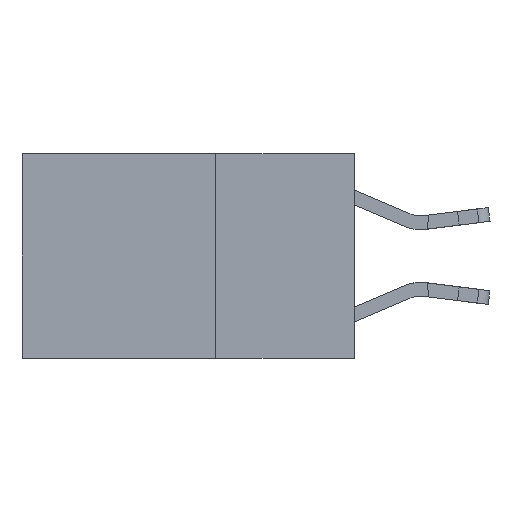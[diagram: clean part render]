
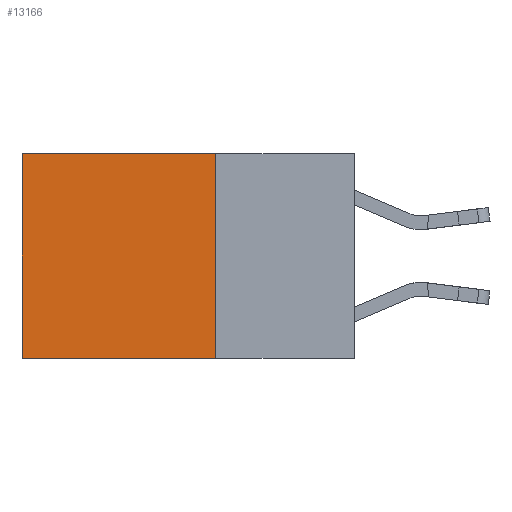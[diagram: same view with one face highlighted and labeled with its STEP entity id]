
A CAD part, left-side view. The second image highlights one B-rep face of the part: STEP entity #13166.
In plain terms, the highlighted planar face has unit normal (-1, 0, 0).
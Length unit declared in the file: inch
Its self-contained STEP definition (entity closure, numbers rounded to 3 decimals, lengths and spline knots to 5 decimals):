
#36 = EDGE_LOOP ( 'NONE', ( #1351, #12212, #3671, #1353 ) ) ;
#276 = FACE_OUTER_BOUND ( 'NONE', #36, .T. ) ;
#510 = DIRECTION ( 'NONE',  ( 0., 0., -1. ) ) ;
#727 = EDGE_CURVE ( 'NONE', #2902, #9760, #1967, .T. ) ;
#980 = VECTOR ( 'NONE', #510, 39.37008 ) ;
#1351 = ORIENTED_EDGE ( 'NONE', *, *, #727, .T. ) ;
#1353 = ORIENTED_EDGE ( 'NONE', *, *, #10405, .T. ) ;
#1362 = CARTESIAN_POINT ( 'NONE',  ( 0.2625, 0.25, 0. ) ) ;
#1462 = VERTEX_POINT ( 'NONE', #5205 ) ;
#1967 = LINE ( 'NONE', #6863, #980 ) ;
#2902 = VERTEX_POINT ( 'NONE', #10292 ) ;
#3411 = EDGE_CURVE ( 'NONE', #1462, #8836, #15473, .T. ) ;
#3662 = DIRECTION ( 'NONE',  ( 1., 0., 0. ) ) ;
#3671 = ORIENTED_EDGE ( 'NONE', *, *, #3411, .F. ) ;
#3880 = CARTESIAN_POINT ( 'NONE',  ( 0.2625, 0.25, -0.37 ) ) ;
#3924 = DIRECTION ( 'NONE',  ( 0., 1., 0. ) ) ;
#5205 = CARTESIAN_POINT ( 'NONE',  ( 0.2625, 0.25, 0. ) ) ;
#5768 = LINE ( 'NONE', #1362, #12105 ) ;
#6618 = CARTESIAN_POINT ( 'NONE',  ( 0.2625, 0.25, 0. ) ) ;
#6775 = DIRECTION ( 'NONE',  ( 0., 1., 0. ) ) ;
#6863 = CARTESIAN_POINT ( 'NONE',  ( 0.2625, 0.6, 0. ) ) ;
#8833 = DIRECTION ( 'NONE',  ( 0., 0., -1. ) ) ;
#8836 = VERTEX_POINT ( 'NONE', #3880 ) ;
#9350 = CARTESIAN_POINT ( 'NONE',  ( 0.2625, 0.6, -0.37 ) ) ;
#9760 = VERTEX_POINT ( 'NONE', #9350 ) ;
#10292 = CARTESIAN_POINT ( 'NONE',  ( 0.2625, 0.6, 0. ) ) ;
#10293 = VECTOR ( 'NONE', #14247, 39.37008 ) ;
#10302 = VECTOR ( 'NONE', #6775, 39.37008 ) ;
#10405 = EDGE_CURVE ( 'NONE', #1462, #2902, #5768, .T. ) ;
#11240 = EDGE_CURVE ( 'NONE', #8836, #9760, #13695, .T. ) ;
#12105 = VECTOR ( 'NONE', #3924, 39.37008 ) ;
#12212 = ORIENTED_EDGE ( 'NONE', *, *, #11240, .F. ) ;
#12481 = PLANE ( 'NONE',  #13456 ) ;
#13091 = CARTESIAN_POINT ( 'NONE',  ( 0.2625, 0.25, -0.37 ) ) ;
#13166 = ADVANCED_FACE ( 'NONE', ( #276 ), #12481, .F. ) ;
#13456 = AXIS2_PLACEMENT_3D ( 'NONE', #16355, #3662, #8833 ) ;
#13695 = LINE ( 'NONE', #13091, #10302 ) ;
#14247 = DIRECTION ( 'NONE',  ( 0., 0., -1. ) ) ;
#15473 = LINE ( 'NONE', #6618, #10293 ) ;
#16355 = CARTESIAN_POINT ( 'NONE',  ( 0.2625, 0.25, 0. ) ) ;
